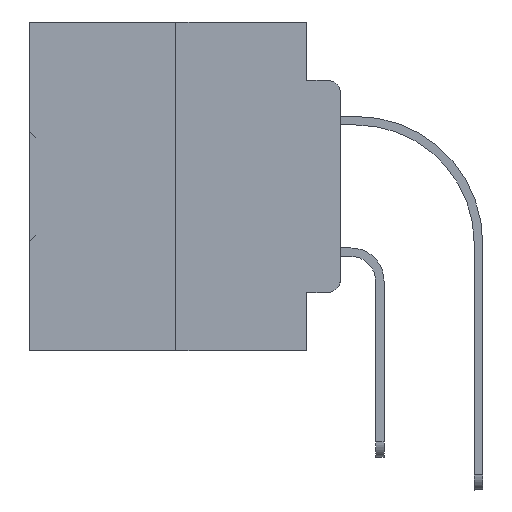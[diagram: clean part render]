
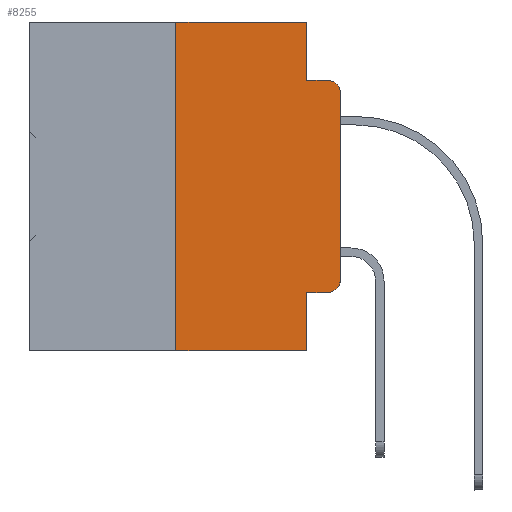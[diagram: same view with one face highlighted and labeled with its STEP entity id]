
A CAD part, left-side view. The second image highlights one B-rep face of the part: STEP entity #8255.
In plain terms, the highlighted planar face has unit normal (-1, 0, 0).
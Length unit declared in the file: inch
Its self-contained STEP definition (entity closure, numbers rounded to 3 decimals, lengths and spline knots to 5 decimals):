
#493 = EDGE_CURVE ( 'NONE', #29935, #35214, #8958, .T. ) ;
#901 = EDGE_CURVE ( 'NONE', #11768, #34793, #10496, .T. ) ;
#926 = LINE ( 'NONE', #16126, #19870 ) ;
#1308 = VERTEX_POINT ( 'NONE', #8855 ) ;
#1762 = EDGE_LOOP ( 'NONE', ( #21351, #34034, #33275, #3898, #4794, #22778, #2460, #33717, #12449, #23278 ) ) ;
#2272 = CARTESIAN_POINT ( 'NONE',  ( 0., 0.473, 0. ) ) ;
#2278 = LINE ( 'NONE', #14054, #3678 ) ;
#2460 = ORIENTED_EDGE ( 'NONE', *, *, #493, .T. ) ;
#3678 = VECTOR ( 'NONE', #26569, 39.37008 ) ;
#3898 = ORIENTED_EDGE ( 'NONE', *, *, #26039, .F. ) ;
#4025 = CIRCLE ( 'NONE', #9844, 0.02 ) ;
#4794 = ORIENTED_EDGE ( 'NONE', *, *, #27315, .F. ) ;
#5270 = CARTESIAN_POINT ( 'NONE',  ( 0., 0.051, 0. ) ) ;
#6104 = DIRECTION ( 'NONE',  ( 0., -1., 0. ) ) ;
#6229 = VECTOR ( 'NONE', #21066, 39.37008 ) ;
#8255 = ADVANCED_FACE ( 'NONE', ( #27182 ), #12215, .F. ) ;
#8822 = EDGE_CURVE ( 'NONE', #38082, #35214, #926, .T. ) ;
#8843 = CARTESIAN_POINT ( 'NONE',  ( 0., 0., -0.1085 ) ) ;
#8855 = CARTESIAN_POINT ( 'NONE',  ( 0., 0.02, -0.4115 ) ) ;
#8958 = LINE ( 'NONE', #33451, #31559 ) ;
#9844 = AXIS2_PLACEMENT_3D ( 'NONE', #12239, #33883, #31037 ) ;
#10295 = DIRECTION ( 'NONE',  ( -1., 0., 0. ) ) ;
#10496 = LINE ( 'NONE', #14783, #29615 ) ;
#10760 = DIRECTION ( 'NONE',  ( 0., -1., 0. ) ) ;
#10922 = DIRECTION ( 'NONE',  ( 0., 0., 1. ) ) ;
#11336 = VERTEX_POINT ( 'NONE', #14597 ) ;
#11768 = VERTEX_POINT ( 'NONE', #34986 ) ;
#12215 = PLANE ( 'NONE',  #34078 ) ;
#12239 = CARTESIAN_POINT ( 'NONE',  ( 0., 0.02, -0.1085 ) ) ;
#12449 = ORIENTED_EDGE ( 'NONE', *, *, #38029, .T. ) ;
#13789 = VECTOR ( 'NONE', #10760, 39.37008 ) ;
#13915 = DIRECTION ( 'NONE',  ( 0., 0., -1. ) ) ;
#14054 = CARTESIAN_POINT ( 'NONE',  ( 0., 0.25, 0. ) ) ;
#14597 = CARTESIAN_POINT ( 'NONE',  ( 0., 0.051, 0. ) ) ;
#14643 = DIRECTION ( 'NONE',  ( 1., 0., 0. ) ) ;
#14783 = CARTESIAN_POINT ( 'NONE',  ( 0., 0.051, -0.0885 ) ) ;
#15486 = EDGE_CURVE ( 'NONE', #20773, #34793, #4025, .T. ) ;
#16126 = CARTESIAN_POINT ( 'NONE',  ( 0., 0.051, 0. ) ) ;
#16737 = CARTESIAN_POINT ( 'NONE',  ( 0., 0.02, -0.3915 ) ) ;
#16792 = EDGE_CURVE ( 'NONE', #39543, #20773, #38434, .T. ) ;
#16800 = CARTESIAN_POINT ( 'NONE',  ( 0., 0.051, -0.4115 ) ) ;
#17397 = CARTESIAN_POINT ( 'NONE',  ( 0., 0.051, -0.4115 ) ) ;
#17654 = DIRECTION ( 'NONE',  ( 0., -1., 0. ) ) ;
#19870 = VECTOR ( 'NONE', #25432, 39.37008 ) ;
#20447 = LINE ( 'NONE', #17397, #13789 ) ;
#20773 = VERTEX_POINT ( 'NONE', #8843 ) ;
#21066 = DIRECTION ( 'NONE',  ( 0., 0., -1. ) ) ;
#21351 = ORIENTED_EDGE ( 'NONE', *, *, #16792, .T. ) ;
#21893 = EDGE_CURVE ( 'NONE', #1308, #39543, #39681, .T. ) ;
#22778 = ORIENTED_EDGE ( 'NONE', *, *, #35906, .F. ) ;
#23278 = ORIENTED_EDGE ( 'NONE', *, *, #21893, .T. ) ;
#23329 = CARTESIAN_POINT ( 'NONE',  ( 0., 0.25, -0.5 ) ) ;
#23509 = VERTEX_POINT ( 'NONE', #24439 ) ;
#24439 = CARTESIAN_POINT ( 'NONE',  ( 0., 0.25, 0. ) ) ;
#25432 = DIRECTION ( 'NONE',  ( 0., 0., -1. ) ) ;
#26039 = EDGE_CURVE ( 'NONE', #11336, #11768, #26938, .T. ) ;
#26569 = DIRECTION ( 'NONE',  ( 0., 0., 1. ) ) ;
#26860 = VECTOR ( 'NONE', #10922, 39.37008 ) ;
#26938 = LINE ( 'NONE', #5270, #6229 ) ;
#27182 = FACE_OUTER_BOUND ( 'NONE', #1762, .T. ) ;
#27315 = EDGE_CURVE ( 'NONE', #23509, #11336, #33053, .T. ) ;
#28726 = CARTESIAN_POINT ( 'NONE',  ( 0., 0.051, -0.5 ) ) ;
#28935 = VECTOR ( 'NONE', #17654, 39.37008 ) ;
#29615 = VECTOR ( 'NONE', #33777, 39.37008 ) ;
#29935 = VERTEX_POINT ( 'NONE', #23329 ) ;
#31037 = DIRECTION ( 'NONE',  ( 0., 0., -1. ) ) ;
#31559 = VECTOR ( 'NONE', #6104, 39.37008 ) ;
#33053 = LINE ( 'NONE', #39137, #28935 ) ;
#33275 = ORIENTED_EDGE ( 'NONE', *, *, #901, .F. ) ;
#33451 = CARTESIAN_POINT ( 'NONE',  ( 0., 0.473, -0.5 ) ) ;
#33717 = ORIENTED_EDGE ( 'NONE', *, *, #8822, .F. ) ;
#33777 = DIRECTION ( 'NONE',  ( 0., -1., 0. ) ) ;
#33880 = AXIS2_PLACEMENT_3D ( 'NONE', #16737, #10295, #13915 ) ;
#33883 = DIRECTION ( 'NONE',  ( -1., 0., 0. ) ) ;
#34034 = ORIENTED_EDGE ( 'NONE', *, *, #15486, .T. ) ;
#34078 = AXIS2_PLACEMENT_3D ( 'NONE', #2272, #14643, #36283 ) ;
#34793 = VERTEX_POINT ( 'NONE', #37541 ) ;
#34986 = CARTESIAN_POINT ( 'NONE',  ( 0., 0.051, -0.0885 ) ) ;
#35214 = VERTEX_POINT ( 'NONE', #28726 ) ;
#35906 = EDGE_CURVE ( 'NONE', #29935, #23509, #2278, .T. ) ;
#36006 = CARTESIAN_POINT ( 'NONE',  ( 0., 0., 0. ) ) ;
#36283 = DIRECTION ( 'NONE',  ( 0., 0., -1. ) ) ;
#37541 = CARTESIAN_POINT ( 'NONE',  ( 0., 0.02, -0.0885 ) ) ;
#38029 = EDGE_CURVE ( 'NONE', #38082, #1308, #20447, .T. ) ;
#38082 = VERTEX_POINT ( 'NONE', #16800 ) ;
#38434 = LINE ( 'NONE', #36006, #26860 ) ;
#39137 = CARTESIAN_POINT ( 'NONE',  ( 0., 0.473, 0. ) ) ;
#39477 = CARTESIAN_POINT ( 'NONE',  ( 0., 0., -0.3915 ) ) ;
#39543 = VERTEX_POINT ( 'NONE', #39477 ) ;
#39681 = CIRCLE ( 'NONE', #33880, 0.02 ) ;
